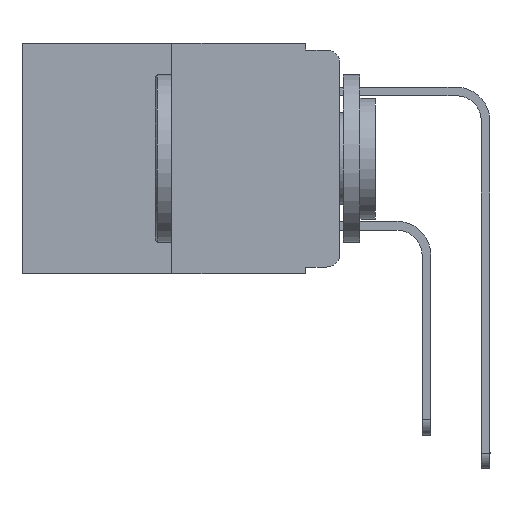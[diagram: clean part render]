
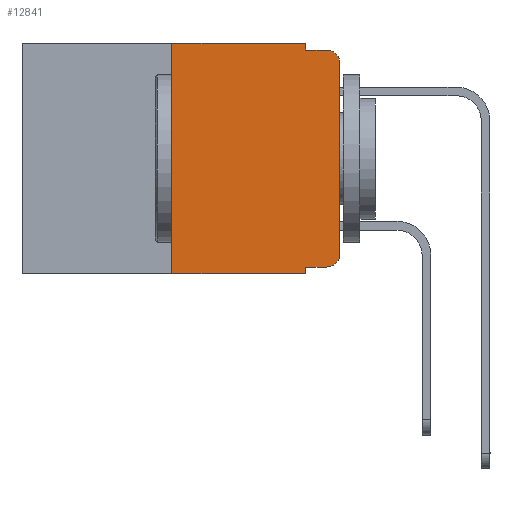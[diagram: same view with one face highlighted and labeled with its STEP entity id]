
A CAD part, left-side view. The second image highlights one B-rep face of the part: STEP entity #12841.
In plain terms, the highlighted planar face has unit normal (-1, 0, 0).
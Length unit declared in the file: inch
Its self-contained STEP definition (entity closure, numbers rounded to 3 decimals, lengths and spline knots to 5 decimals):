
#63 = EDGE_CURVE ( 'NONE', #3208, #5194, #1141, .T. ) ;
#123 = DIRECTION ( 'NONE',  ( 0., 0., -1. ) ) ;
#221 = VERTEX_POINT ( 'NONE', #12980 ) ;
#225 = EDGE_CURVE ( 'NONE', #8865, #8925, #13055, .T. ) ;
#227 = DIRECTION ( 'NONE',  ( 0., 0., -1. ) ) ;
#414 = VECTOR ( 'NONE', #227, 39.37008 ) ;
#521 = CARTESIAN_POINT ( 'NONE',  ( 0., 0.02, -0.01 ) ) ;
#714 = DIRECTION ( 'NONE',  ( 0., -1., 0. ) ) ;
#868 = ORIENTED_EDGE ( 'NONE', *, *, #5472, .F. ) ;
#943 = LINE ( 'NONE', #12535, #3985 ) ;
#1141 = CIRCLE ( 'NONE', #6107, 0.02 ) ;
#1246 = VECTOR ( 'NONE', #7622, 39.37008 ) ;
#1299 = LINE ( 'NONE', #8370, #1468 ) ;
#1468 = VECTOR ( 'NONE', #7128, 39.37008 ) ;
#1577 = EDGE_CURVE ( 'NONE', #4480, #6072, #13287, .T. ) ;
#1621 = CARTESIAN_POINT ( 'NONE',  ( 0., 0.051, -0.343 ) ) ;
#2447 = DIRECTION ( 'NONE',  ( -1., 0., 0. ) ) ;
#2481 = DIRECTION ( 'NONE',  ( 1., 0., 0. ) ) ;
#2507 = DIRECTION ( 'NONE',  ( 0., 0., 1. ) ) ;
#2536 = DIRECTION ( 'NONE',  ( 0., -1., 0. ) ) ;
#2893 = EDGE_CURVE ( 'NONE', #8865, #12116, #12209, .T. ) ;
#3061 = LINE ( 'NONE', #12517, #6832 ) ;
#3208 = VERTEX_POINT ( 'NONE', #3966 ) ;
#3393 = ORIENTED_EDGE ( 'NONE', *, *, #2893, .T. ) ;
#3606 = EDGE_CURVE ( 'NONE', #221, #3208, #1299, .T. ) ;
#3861 = VECTOR ( 'NONE', #2507, 39.37008 ) ;
#3966 = CARTESIAN_POINT ( 'NONE',  ( 0., 0., -0.03 ) ) ;
#3985 = VECTOR ( 'NONE', #9317, 39.37008 ) ;
#4289 = ORIENTED_EDGE ( 'NONE', *, *, #14972, .T. ) ;
#4410 = ORIENTED_EDGE ( 'NONE', *, *, #11235, .F. ) ;
#4480 = VERTEX_POINT ( 'NONE', #4673 ) ;
#4673 = CARTESIAN_POINT ( 'NONE',  ( 0., 0.25, -0.343 ) ) ;
#4982 = CARTESIAN_POINT ( 'NONE',  ( 0., 0.25, 0. ) ) ;
#5031 = ORIENTED_EDGE ( 'NONE', *, *, #1577, .F. ) ;
#5194 = VERTEX_POINT ( 'NONE', #521 ) ;
#5431 = CARTESIAN_POINT ( 'NONE',  ( 0., 0.25, 0. ) ) ;
#5472 = EDGE_CURVE ( 'NONE', #6072, #10124, #6882, .T. ) ;
#5911 = CARTESIAN_POINT ( 'NONE',  ( 0., 0.051, 0. ) ) ;
#5966 = VECTOR ( 'NONE', #6042, 39.37008 ) ;
#6042 = DIRECTION ( 'NONE',  ( 0., -1., 0. ) ) ;
#6072 = VERTEX_POINT ( 'NONE', #5431 ) ;
#6107 = AXIS2_PLACEMENT_3D ( 'NONE', #7780, #12520, #6695 ) ;
#6542 = CARTESIAN_POINT ( 'NONE',  ( 0., 0.02, -0.333 ) ) ;
#6695 = DIRECTION ( 'NONE',  ( 0., 0., -1. ) ) ;
#6832 = VECTOR ( 'NONE', #714, 39.37008 ) ;
#6882 = LINE ( 'NONE', #14343, #8332 ) ;
#7128 = DIRECTION ( 'NONE',  ( 0., 0., 1. ) ) ;
#7622 = DIRECTION ( 'NONE',  ( 0., -1., 0. ) ) ;
#7780 = CARTESIAN_POINT ( 'NONE',  ( 0., 0.02, -0.03 ) ) ;
#8332 = VECTOR ( 'NONE', #2536, 39.37008 ) ;
#8351 = ORIENTED_EDGE ( 'NONE', *, *, #3606, .T. ) ;
#8370 = CARTESIAN_POINT ( 'NONE',  ( 0., 0., 0. ) ) ;
#8524 = PLANE ( 'NONE',  #14152 ) ;
#8565 = DIRECTION ( 'NONE',  ( 0., 0., -1. ) ) ;
#8644 = ORIENTED_EDGE ( 'NONE', *, *, #12860, .F. ) ;
#8865 = VERTEX_POINT ( 'NONE', #9397 ) ;
#8925 = VERTEX_POINT ( 'NONE', #1621 ) ;
#9317 = DIRECTION ( 'NONE',  ( 0., 0., -1. ) ) ;
#9397 = CARTESIAN_POINT ( 'NONE',  ( 0., 0.051, -0.333 ) ) ;
#9941 = EDGE_CURVE ( 'NONE', #4480, #8925, #3061, .T. ) ;
#10120 = ORIENTED_EDGE ( 'NONE', *, *, #63, .T. ) ;
#10124 = VERTEX_POINT ( 'NONE', #5911 ) ;
#10804 = CARTESIAN_POINT ( 'NONE',  ( 0., 0.051, 0. ) ) ;
#10900 = CARTESIAN_POINT ( 'NONE',  ( 0., 0.02, -0.313 ) ) ;
#11235 = EDGE_CURVE ( 'NONE', #10124, #11808, #943, .T. ) ;
#11807 = AXIS2_PLACEMENT_3D ( 'NONE', #10900, #2447, #8565 ) ;
#11808 = VERTEX_POINT ( 'NONE', #14600 ) ;
#12045 = ORIENTED_EDGE ( 'NONE', *, *, #225, .F. ) ;
#12098 = LINE ( 'NONE', #14441, #5966 ) ;
#12116 = VERTEX_POINT ( 'NONE', #6542 ) ;
#12209 = LINE ( 'NONE', #13523, #1246 ) ;
#12329 = ORIENTED_EDGE ( 'NONE', *, *, #9941, .T. ) ;
#12517 = CARTESIAN_POINT ( 'NONE',  ( 0., 0.473, -0.343 ) ) ;
#12520 = DIRECTION ( 'NONE',  ( -1., 0., 0. ) ) ;
#12535 = CARTESIAN_POINT ( 'NONE',  ( 0., 0.051, 0. ) ) ;
#12841 = ADVANCED_FACE ( 'NONE', ( #14509 ), #8524, .F. ) ;
#12860 = EDGE_CURVE ( 'NONE', #11808, #5194, #12098, .T. ) ;
#12980 = CARTESIAN_POINT ( 'NONE',  ( 0., 0., -0.313 ) ) ;
#13055 = LINE ( 'NONE', #10804, #414 ) ;
#13190 = CARTESIAN_POINT ( 'NONE',  ( 0., 0.473, 0. ) ) ;
#13287 = LINE ( 'NONE', #4982, #3861 ) ;
#13292 = CIRCLE ( 'NONE', #11807, 0.02 ) ;
#13523 = CARTESIAN_POINT ( 'NONE',  ( 0., 0.051, -0.333 ) ) ;
#14152 = AXIS2_PLACEMENT_3D ( 'NONE', #13190, #2481, #123 ) ;
#14244 = EDGE_LOOP ( 'NONE', ( #8351, #10120, #8644, #4410, #868, #5031, #12329, #12045, #3393, #4289 ) ) ;
#14343 = CARTESIAN_POINT ( 'NONE',  ( 0., 0.473, 0. ) ) ;
#14441 = CARTESIAN_POINT ( 'NONE',  ( 0., 0.051, -0.01 ) ) ;
#14509 = FACE_OUTER_BOUND ( 'NONE', #14244, .T. ) ;
#14600 = CARTESIAN_POINT ( 'NONE',  ( 0., 0.051, -0.01 ) ) ;
#14972 = EDGE_CURVE ( 'NONE', #12116, #221, #13292, .T. ) ;
